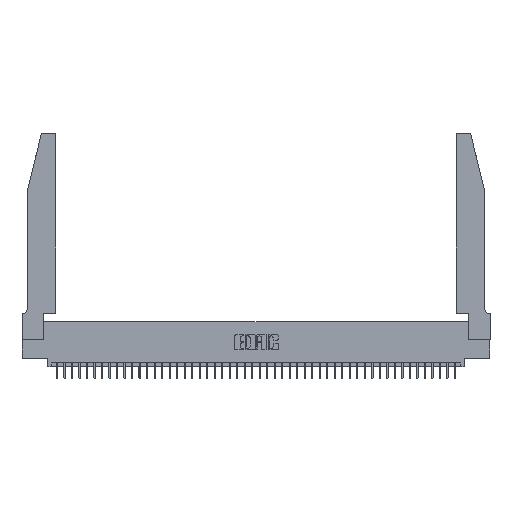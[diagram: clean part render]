
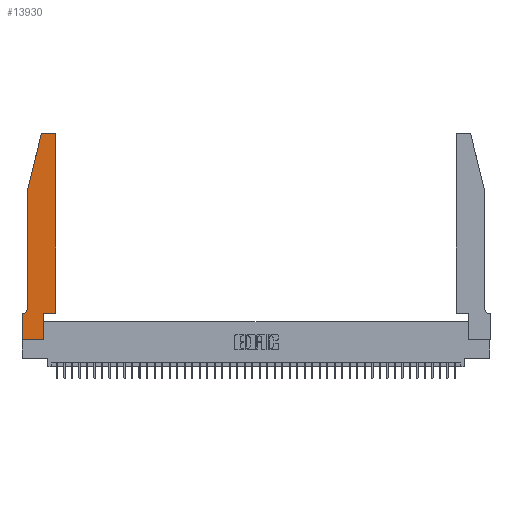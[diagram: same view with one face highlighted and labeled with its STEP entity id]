
A CAD part, top view. The second image highlights one B-rep face of the part: STEP entity #13930.
In plain terms, the highlighted planar face has unit normal (0, 0, 1).
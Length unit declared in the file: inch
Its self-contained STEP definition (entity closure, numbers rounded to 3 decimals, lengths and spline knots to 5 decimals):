
#585 = CARTESIAN_POINT ( 'NONE',  ( 0.0755, 0.35, 0.37 ) ) ;
#1408 = CARTESIAN_POINT ( 'NONE',  ( 0.284, 2.72, 0.37 ) ) ;
#2126 = DIRECTION ( 'NONE',  ( 0., 0., -1. ) ) ;
#2434 = CARTESIAN_POINT ( 'NONE',  ( 0.284, 2.75, 0.37 ) ) ;
#2727 = ORIENTED_EDGE ( 'NONE', *, *, #45364, .T. ) ;
#2792 = VERTEX_POINT ( 'NONE', #15424 ) ;
#2809 = CARTESIAN_POINT ( 'NONE',  ( 0., 0., 0.37 ) ) ;
#4004 = DIRECTION ( 'NONE',  ( -0.239, -0.971, 0. ) ) ;
#4184 = CARTESIAN_POINT ( 'NONE',  ( 0., 0., 0.37 ) ) ;
#4970 = DIRECTION ( 'NONE',  ( 1., 0., 0. ) ) ;
#5113 = VECTOR ( 'NONE', #16181, 39.37008 ) ;
#6340 = LINE ( 'NONE', #32334, #33436 ) ;
#6409 = LINE ( 'NONE', #585, #14781 ) ;
#6439 = EDGE_CURVE ( 'NONE', #24905, #2792, #6340, .T. ) ;
#6967 = CARTESIAN_POINT ( 'NONE',  ( 0.4505, 0.35, 0.37 ) ) ;
#6968 = ORIENTED_EDGE ( 'NONE', *, *, #33691, .T. ) ;
#7733 = DIRECTION ( 'NONE',  ( 0., -1., 0. ) ) ;
#7893 = CIRCLE ( 'NONE', #40619, 0.03 ) ;
#8004 = ORIENTED_EDGE ( 'NONE', *, *, #18662, .T. ) ;
#9232 = PLANE ( 'NONE',  #35776 ) ;
#9438 = ORIENTED_EDGE ( 'NONE', *, *, #41888, .T. ) ;
#10021 = CARTESIAN_POINT ( 'NONE',  ( 0.2865, 0., 0.37 ) ) ;
#10585 = DIRECTION ( 'NONE',  ( 0., 1., 0. ) ) ;
#12851 = CARTESIAN_POINT ( 'NONE',  ( 0., 0.35, 0.37 ) ) ;
#12873 = CARTESIAN_POINT ( 'NONE',  ( 0.2865, 0.35, 0.37 ) ) ;
#13930 = ADVANCED_FACE ( 'NONE', ( #14873 ), #9232, .T. ) ;
#14144 = ORIENTED_EDGE ( 'NONE', *, *, #15812, .T. ) ;
#14230 = AXIS2_PLACEMENT_3D ( 'NONE', #1408, #26222, #4970 ) ;
#14552 = LINE ( 'NONE', #6967, #22823 ) ;
#14662 = CARTESIAN_POINT ( 'NONE',  ( 0.0055, 0.35, 0.37 ) ) ;
#14781 = VECTOR ( 'NONE', #25389, 39.37008 ) ;
#14873 = FACE_OUTER_BOUND ( 'NONE', #15692, .T. ) ;
#15284 = VERTEX_POINT ( 'NONE', #14662 ) ;
#15424 = CARTESIAN_POINT ( 'NONE',  ( 0.0755, 2., 0.37 ) ) ;
#15666 = CARTESIAN_POINT ( 'NONE',  ( 0.4505, 0.35, 0.37 ) ) ;
#15692 = EDGE_LOOP ( 'NONE', ( #30881, #9438, #20226, #14144, #20332, #8004, #31664, #43243, #28904, #6968, #2727, #32722 ) ) ;
#15812 = EDGE_CURVE ( 'NONE', #2792, #30350, #22485, .T. ) ;
#16096 = DIRECTION ( 'NONE',  ( 0., 0., 1. ) ) ;
#16150 = VERTEX_POINT ( 'NONE', #15666 ) ;
#16181 = DIRECTION ( 'NONE',  ( -1., 0., 0. ) ) ;
#16406 = DIRECTION ( 'NONE',  ( 0., 0., 1. ) ) ;
#17957 = CARTESIAN_POINT ( 'NONE',  ( 0.4505, 0.35, 0.37 ) ) ;
#18662 = EDGE_CURVE ( 'NONE', #15284, #44645, #6409, .T. ) ;
#20226 = ORIENTED_EDGE ( 'NONE', *, *, #6439, .T. ) ;
#20332 = ORIENTED_EDGE ( 'NONE', *, *, #37826, .T. ) ;
#20525 = DIRECTION ( 'NONE',  ( 1., 0., 0. ) ) ;
#21419 = CARTESIAN_POINT ( 'NONE',  ( 0.25487, 2.72718, 0.37 ) ) ;
#22326 = VERTEX_POINT ( 'NONE', #38732 ) ;
#22485 = LINE ( 'NONE', #45558, #41184 ) ;
#22823 = VECTOR ( 'NONE', #10585, 39.37008 ) ;
#22896 = CIRCLE ( 'NONE', #24779, 0.07 ) ;
#23032 = LINE ( 'NONE', #12873, #31311 ) ;
#23402 = CARTESIAN_POINT ( 'NONE',  ( 0.0055, 0.42, 0.37 ) ) ;
#23721 = VECTOR ( 'NONE', #7733, 39.37008 ) ;
#24158 = CARTESIAN_POINT ( 'NONE',  ( 0., 0., 0.37 ) ) ;
#24503 = DIRECTION ( 'NONE',  ( 0., -1., 0. ) ) ;
#24779 = AXIS2_PLACEMENT_3D ( 'NONE', #23402, #2126, #26965 ) ;
#24905 = VERTEX_POINT ( 'NONE', #21419 ) ;
#25389 = DIRECTION ( 'NONE',  ( -1., 0., 0. ) ) ;
#25824 = CIRCLE ( 'NONE', #14230, 0.03 ) ;
#26222 = DIRECTION ( 'NONE',  ( 0., 0., 1. ) ) ;
#26251 = CARTESIAN_POINT ( 'NONE',  ( 0.4205, 2.75, 0.37 ) ) ;
#26965 = DIRECTION ( 'NONE',  ( -1., 0., 0. ) ) ;
#27233 = CARTESIAN_POINT ( 'NONE',  ( 0.2865, 0.35, 0.37 ) ) ;
#27704 = LINE ( 'NONE', #17957, #44116 ) ;
#28904 = ORIENTED_EDGE ( 'NONE', *, *, #28971, .T. ) ;
#28971 = EDGE_CURVE ( 'NONE', #31657, #38624, #23032, .T. ) ;
#29174 = VERTEX_POINT ( 'NONE', #2434 ) ;
#30209 = CARTESIAN_POINT ( 'NONE',  ( 0.2605, 2.75, 0.37 ) ) ;
#30337 = EDGE_CURVE ( 'NONE', #40983, #29174, #34469, .T. ) ;
#30350 = VERTEX_POINT ( 'NONE', #44325 ) ;
#30881 = ORIENTED_EDGE ( 'NONE', *, *, #30337, .T. ) ;
#31311 = VECTOR ( 'NONE', #44419, 39.37008 ) ;
#31468 = EDGE_CURVE ( 'NONE', #22326, #40983, #7893, .T. ) ;
#31657 = VERTEX_POINT ( 'NONE', #10021 ) ;
#31664 = ORIENTED_EDGE ( 'NONE', *, *, #34507, .T. ) ;
#32334 = CARTESIAN_POINT ( 'NONE',  ( 0.0755, 2., 0.37 ) ) ;
#32722 = ORIENTED_EDGE ( 'NONE', *, *, #31468, .T. ) ;
#33436 = VECTOR ( 'NONE', #4004, 39.37008 ) ;
#33691 = EDGE_CURVE ( 'NONE', #38624, #16150, #27704, .T. ) ;
#34469 = LINE ( 'NONE', #30209, #5113 ) ;
#34507 = EDGE_CURVE ( 'NONE', #44645, #38034, #42404, .T. ) ;
#35337 = DIRECTION ( 'NONE',  ( 1., 0., 0. ) ) ;
#35776 = AXIS2_PLACEMENT_3D ( 'NONE', #12851, #16406, #41016 ) ;
#37030 = LINE ( 'NONE', #2809, #44194 ) ;
#37151 = CARTESIAN_POINT ( 'NONE',  ( 0.4205, 2.72, 0.37 ) ) ;
#37826 = EDGE_CURVE ( 'NONE', #30350, #15284, #22896, .T. ) ;
#38034 = VERTEX_POINT ( 'NONE', #24158 ) ;
#38624 = VERTEX_POINT ( 'NONE', #27233 ) ;
#38732 = CARTESIAN_POINT ( 'NONE',  ( 0.4505, 2.72, 0.37 ) ) ;
#39308 = EDGE_CURVE ( 'NONE', #38034, #31657, #37030, .T. ) ;
#40619 = AXIS2_PLACEMENT_3D ( 'NONE', #37151, #16096, #40709 ) ;
#40709 = DIRECTION ( 'NONE',  ( 1., 0., 0. ) ) ;
#40983 = VERTEX_POINT ( 'NONE', #26251 ) ;
#41003 = CARTESIAN_POINT ( 'NONE',  ( 0., 0.35, 0.37 ) ) ;
#41016 = DIRECTION ( 'NONE',  ( 1., 0., 0. ) ) ;
#41184 = VECTOR ( 'NONE', #24503, 39.37008 ) ;
#41888 = EDGE_CURVE ( 'NONE', #29174, #24905, #25824, .T. ) ;
#42404 = LINE ( 'NONE', #4184, #23721 ) ;
#43243 = ORIENTED_EDGE ( 'NONE', *, *, #39308, .T. ) ;
#44116 = VECTOR ( 'NONE', #35337, 39.37008 ) ;
#44194 = VECTOR ( 'NONE', #20525, 39.37008 ) ;
#44325 = CARTESIAN_POINT ( 'NONE',  ( 0.0755, 0.42, 0.37 ) ) ;
#44419 = DIRECTION ( 'NONE',  ( 0., 1., 0. ) ) ;
#44645 = VERTEX_POINT ( 'NONE', #41003 ) ;
#45364 = EDGE_CURVE ( 'NONE', #16150, #22326, #14552, .T. ) ;
#45558 = CARTESIAN_POINT ( 'NONE',  ( 0.0755, 2., 0.37 ) ) ;
